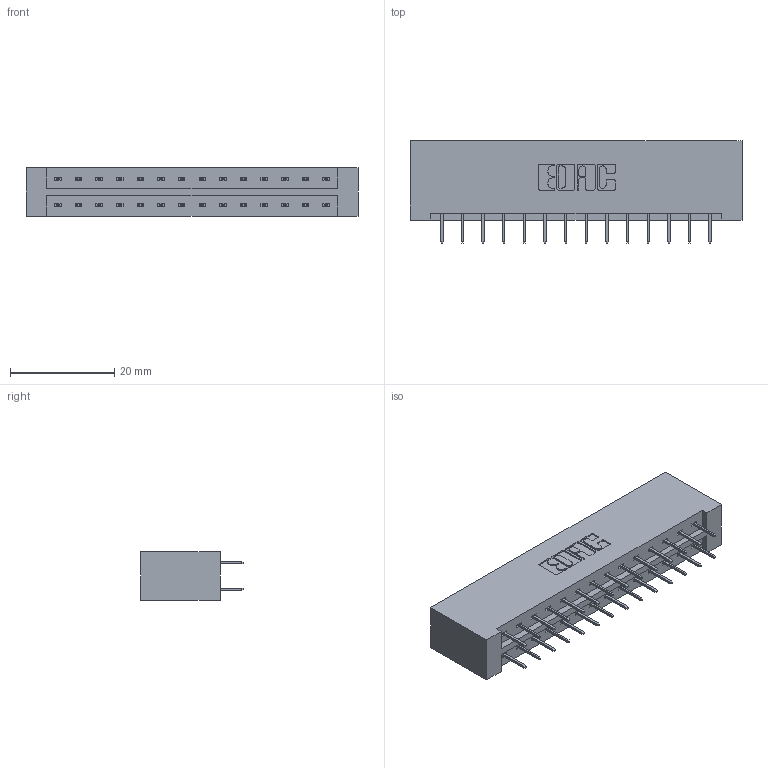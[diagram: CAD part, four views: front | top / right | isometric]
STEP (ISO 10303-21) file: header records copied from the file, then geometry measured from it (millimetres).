
FILE_DESCRIPTION (( 'STEP AP203' ), '1' );
FILE_NAME ('833-028-524-201.STEP', '2020-06-02T08:17:47', ( '' ), ( '' ), 'SwSTEP 2.0', 'SolidWorks 2020', '' );
FILE_SCHEMA (( 'CONFIG_CONTROL_DESIGN' ));
Length unit declared in the file: inch
Products named in the file (3): 833 Part_Lugless; 833-028-524-201; 345-292-001_345-293-124
Assembly tree (29 placements, depth 2):
  833-028-524-201
    833 Part_Lugless
    345-292-001_345-293-124  x28
Bounding box: 63.73 x 19.69 x 9.4 mm (x, y, z)
Volume: 6834.3 mm3; surface area: 7676.2 mm2
Topology: 29 solids, 29 shells, 1674 faces, 4739 edges, 3046 vertices
Faces by surface type: plane 1242, cylinder 432
Entity records: 12425 total; most frequent: CARTESIAN_POINT 2090, ORIENTED_EDGE 2026, DIRECTION 1829, EDGE_CURVE 1013, VECTOR 897, LINE 897, VERTEX_POINT 670, AXIS2_PLACEMENT_3D 466
